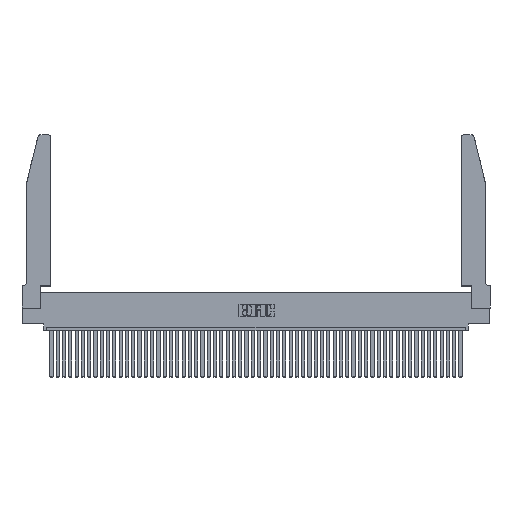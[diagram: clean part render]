
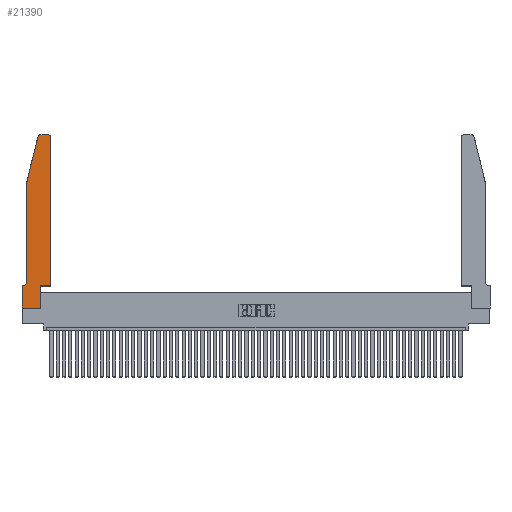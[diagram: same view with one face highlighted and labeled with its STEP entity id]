
A CAD part, top view. The second image highlights one B-rep face of the part: STEP entity #21390.
In plain terms, the highlighted planar face has unit normal (0, 0, 1).
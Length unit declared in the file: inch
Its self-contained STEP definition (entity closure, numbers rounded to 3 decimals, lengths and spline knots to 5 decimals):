
#860 = DIRECTION ( 'NONE',  ( 1., 0., 0. ) ) ;
#1147 = CIRCLE ( 'NONE', #8805, 0.03 ) ;
#1171 = ORIENTED_EDGE ( 'NONE', *, *, #43245, .T. ) ;
#1588 = CARTESIAN_POINT ( 'NONE',  ( 0., 0.35, 0.37 ) ) ;
#2067 = AXIS2_PLACEMENT_3D ( 'NONE', #32320, #47843, #36429 ) ;
#2399 = CARTESIAN_POINT ( 'NONE',  ( 0.2865, 0., 0.37 ) ) ;
#2666 = VERTEX_POINT ( 'NONE', #36778 ) ;
#4048 = LINE ( 'NONE', #29226, #34412 ) ;
#4160 = VERTEX_POINT ( 'NONE', #15394 ) ;
#4564 = CARTESIAN_POINT ( 'NONE',  ( 0.0755, 2., 0.37 ) ) ;
#5051 = LINE ( 'NONE', #49902, #47093 ) ;
#6466 = ORIENTED_EDGE ( 'NONE', *, *, #34716, .T. ) ;
#6528 = VERTEX_POINT ( 'NONE', #30775 ) ;
#8779 = CARTESIAN_POINT ( 'NONE',  ( 0.4505, 0.35, 0.37 ) ) ;
#8805 = AXIS2_PLACEMENT_3D ( 'NONE', #28998, #40830, #17297 ) ;
#8835 = CARTESIAN_POINT ( 'NONE',  ( 0.4205, 2.72, 0.37 ) ) ;
#8943 = CARTESIAN_POINT ( 'NONE',  ( 0.2605, 2.75, 0.37 ) ) ;
#9507 = LINE ( 'NONE', #10971, #23225 ) ;
#9730 = CARTESIAN_POINT ( 'NONE',  ( 0.4505, 2.72, 0.37 ) ) ;
#10971 = CARTESIAN_POINT ( 'NONE',  ( 0.0755, 0.35, 0.37 ) ) ;
#11697 = VECTOR ( 'NONE', #36582, 39.37008 ) ;
#12621 = EDGE_CURVE ( 'NONE', #27700, #35369, #22564, .T. ) ;
#12979 = EDGE_CURVE ( 'NONE', #32835, #23211, #15679, .T. ) ;
#13048 = VERTEX_POINT ( 'NONE', #1588 ) ;
#13327 = CARTESIAN_POINT ( 'NONE',  ( 0.0055, 0.42, 0.37 ) ) ;
#14030 = VERTEX_POINT ( 'NONE', #14130 ) ;
#14130 = CARTESIAN_POINT ( 'NONE',  ( 0.2865, 0.35, 0.37 ) ) ;
#14890 = VERTEX_POINT ( 'NONE', #16017 ) ;
#15337 = FACE_OUTER_BOUND ( 'NONE', #16922, .T. ) ;
#15394 = CARTESIAN_POINT ( 'NONE',  ( 0.0755, 0.42, 0.37 ) ) ;
#15679 = CIRCLE ( 'NONE', #41833, 0.03 ) ;
#15964 = DIRECTION ( 'NONE',  ( -0.239, -0.971, 0. ) ) ;
#16017 = CARTESIAN_POINT ( 'NONE',  ( 0.4505, 0.35, 0.37 ) ) ;
#16486 = DIRECTION ( 'NONE',  ( 0., 1., 0. ) ) ;
#16922 = EDGE_LOOP ( 'NONE', ( #1171, #33378, #34250, #48793, #41231, #42235, #6466, #22177, #27924, #26061, #22209, #34151 ) ) ;
#17297 = DIRECTION ( 'NONE',  ( 1., 0., 0. ) ) ;
#21276 = EDGE_CURVE ( 'NONE', #43388, #14030, #28900, .T. ) ;
#21390 = ADVANCED_FACE ( 'NONE', ( #15337 ), #27996, .T. ) ;
#22025 = CIRCLE ( 'NONE', #49618, 0.07 ) ;
#22177 = ORIENTED_EDGE ( 'NONE', *, *, #38786, .T. ) ;
#22209 = ORIENTED_EDGE ( 'NONE', *, *, #29166, .T. ) ;
#22473 = CARTESIAN_POINT ( 'NONE',  ( 0.0055, 0.35, 0.37 ) ) ;
#22564 = LINE ( 'NONE', #50807, #23768 ) ;
#22882 = CARTESIAN_POINT ( 'NONE',  ( 0.0755, 2., 0.37 ) ) ;
#23211 = VERTEX_POINT ( 'NONE', #27799 ) ;
#23225 = VECTOR ( 'NONE', #47185, 39.37008 ) ;
#23768 = VECTOR ( 'NONE', #15964, 39.37008 ) ;
#25208 = VECTOR ( 'NONE', #16486, 39.37008 ) ;
#25303 = CARTESIAN_POINT ( 'NONE',  ( 0.25487, 2.72718, 0.37 ) ) ;
#26061 = ORIENTED_EDGE ( 'NONE', *, *, #32827, .T. ) ;
#26913 = VECTOR ( 'NONE', #45757, 39.37008 ) ;
#27700 = VERTEX_POINT ( 'NONE', #25303 ) ;
#27799 = CARTESIAN_POINT ( 'NONE',  ( 0.4205, 2.75, 0.37 ) ) ;
#27924 = ORIENTED_EDGE ( 'NONE', *, *, #21276, .T. ) ;
#27996 = PLANE ( 'NONE',  #2067 ) ;
#28552 = DIRECTION ( 'NONE',  ( 1., 0., 0. ) ) ;
#28900 = LINE ( 'NONE', #50893, #25208 ) ;
#28998 = CARTESIAN_POINT ( 'NONE',  ( 0.284, 2.72, 0.37 ) ) ;
#29166 = EDGE_CURVE ( 'NONE', #14890, #32835, #4048, .T. ) ;
#29211 = DIRECTION ( 'NONE',  ( 0., 0., -1. ) ) ;
#29226 = CARTESIAN_POINT ( 'NONE',  ( 0.4505, 0.35, 0.37 ) ) ;
#30079 = EDGE_CURVE ( 'NONE', #41499, #13048, #9507, .T. ) ;
#30775 = CARTESIAN_POINT ( 'NONE',  ( 0., 0., 0.37 ) ) ;
#32320 = CARTESIAN_POINT ( 'NONE',  ( 0., 0.35, 0.37 ) ) ;
#32748 = LINE ( 'NONE', #8779, #49441 ) ;
#32827 = EDGE_CURVE ( 'NONE', #14030, #14890, #32748, .T. ) ;
#32835 = VERTEX_POINT ( 'NONE', #9730 ) ;
#33378 = ORIENTED_EDGE ( 'NONE', *, *, #43292, .T. ) ;
#34151 = ORIENTED_EDGE ( 'NONE', *, *, #12979, .T. ) ;
#34250 = ORIENTED_EDGE ( 'NONE', *, *, #12621, .T. ) ;
#34253 = EDGE_CURVE ( 'NONE', #35369, #4160, #36920, .T. ) ;
#34412 = VECTOR ( 'NONE', #40880, 39.37008 ) ;
#34716 = EDGE_CURVE ( 'NONE', #13048, #6528, #5051, .T. ) ;
#35201 = LINE ( 'NONE', #8943, #11697 ) ;
#35369 = VERTEX_POINT ( 'NONE', #22882 ) ;
#36429 = DIRECTION ( 'NONE',  ( 1., 0., 0. ) ) ;
#36482 = DIRECTION ( 'NONE',  ( 0., 0., 1. ) ) ;
#36582 = DIRECTION ( 'NONE',  ( -1., 0., 0. ) ) ;
#36778 = CARTESIAN_POINT ( 'NONE',  ( 0.284, 2.75, 0.37 ) ) ;
#36920 = LINE ( 'NONE', #4564, #44303 ) ;
#37881 = CARTESIAN_POINT ( 'NONE',  ( 0., 0., 0.37 ) ) ;
#38342 = DIRECTION ( 'NONE',  ( 0., -1., 0. ) ) ;
#38786 = EDGE_CURVE ( 'NONE', #6528, #43388, #41004, .T. ) ;
#40830 = DIRECTION ( 'NONE',  ( 0., 0., 1. ) ) ;
#40880 = DIRECTION ( 'NONE',  ( 0., 1., 0. ) ) ;
#41004 = LINE ( 'NONE', #37881, #26913 ) ;
#41231 = ORIENTED_EDGE ( 'NONE', *, *, #47419, .T. ) ;
#41499 = VERTEX_POINT ( 'NONE', #22473 ) ;
#41833 = AXIS2_PLACEMENT_3D ( 'NONE', #8835, #36482, #28552 ) ;
#42235 = ORIENTED_EDGE ( 'NONE', *, *, #30079, .T. ) ;
#43245 = EDGE_CURVE ( 'NONE', #23211, #2666, #35201, .T. ) ;
#43292 = EDGE_CURVE ( 'NONE', #2666, #27700, #1147, .T. ) ;
#43388 = VERTEX_POINT ( 'NONE', #2399 ) ;
#44303 = VECTOR ( 'NONE', #47622, 39.37008 ) ;
#44349 = DIRECTION ( 'NONE',  ( -1., 0., 0. ) ) ;
#45757 = DIRECTION ( 'NONE',  ( 1., 0., 0. ) ) ;
#47093 = VECTOR ( 'NONE', #38342, 39.37008 ) ;
#47185 = DIRECTION ( 'NONE',  ( -1., 0., 0. ) ) ;
#47419 = EDGE_CURVE ( 'NONE', #4160, #41499, #22025, .T. ) ;
#47622 = DIRECTION ( 'NONE',  ( 0., -1., 0. ) ) ;
#47843 = DIRECTION ( 'NONE',  ( 0., 0., 1. ) ) ;
#48793 = ORIENTED_EDGE ( 'NONE', *, *, #34253, .T. ) ;
#49441 = VECTOR ( 'NONE', #860, 39.37008 ) ;
#49618 = AXIS2_PLACEMENT_3D ( 'NONE', #13327, #29211, #44349 ) ;
#49902 = CARTESIAN_POINT ( 'NONE',  ( 0., 0., 0.37 ) ) ;
#50807 = CARTESIAN_POINT ( 'NONE',  ( 0.0755, 2., 0.37 ) ) ;
#50893 = CARTESIAN_POINT ( 'NONE',  ( 0.2865, 0.35, 0.37 ) ) ;
